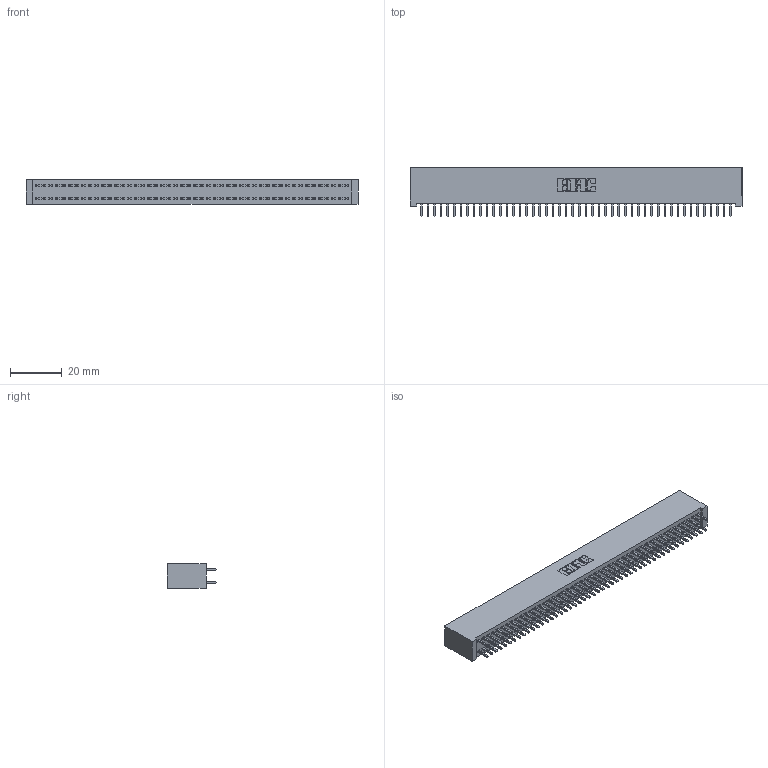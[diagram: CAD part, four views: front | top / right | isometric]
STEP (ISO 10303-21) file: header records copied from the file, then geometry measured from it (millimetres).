
FILE_DESCRIPTION (( 'STEP AP203' ), '1' );
FILE_NAME ('342-096-521-201.STEP', '2018-08-14T02:58:36', ( '' ), ( '' ), 'SwSTEP 2.0', 'SolidWorks 2016', '' );
FILE_SCHEMA (( 'CONFIG_CONTROL_DESIGN' ));
Length unit declared in the file: inch
Products named in the file (3): 342 Part_Lugless; 345-292-001_345-293-121; 342-096-521-201
Assembly tree (97 placements, depth 2):
  342-096-521-201
    342 Part_Lugless
    345-292-001_345-293-121  x96
Bounding box: 128.17 x 19.06 x 9.4 mm (x, y, z)
Volume: 11944.6 mm3; surface area: 19771.7 mm2
Topology: 97 solids, 97 shells, 5094 faces, 15155 edges, 9974 vertices
Faces by surface type: plane 3518, cylinder 1576
Entity records: 29713 total; most frequent: CARTESIAN_POINT 4914, ORIENTED_EDGE 4850, DIRECTION 4181, EDGE_CURVE 2425, VECTOR 2305, LINE 2305, VERTEX_POINT 1614, AXIS2_PLACEMENT_3D 938
